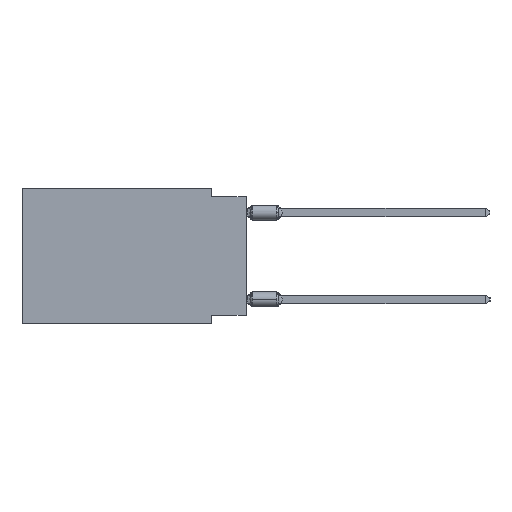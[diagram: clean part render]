
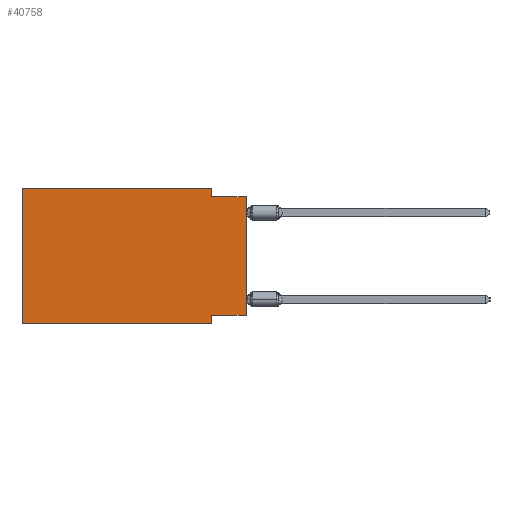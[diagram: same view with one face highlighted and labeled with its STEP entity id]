
A CAD part, left-side view. The second image highlights one B-rep face of the part: STEP entity #40758.
In plain terms, the highlighted planar face has unit normal (-1, 0, 0).
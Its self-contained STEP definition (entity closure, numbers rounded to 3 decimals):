
#18 = CARTESIAN_POINT ( 'NONE',  ( 0., 16.383, 0. ) ) ;
#158 = ORIENTED_EDGE ( 'NONE', *, *, #26595, .F. ) ;
#1688 = VERTEX_POINT ( 'NONE', #26304 ) ;
#2067 = ORIENTED_EDGE ( 'NONE', *, *, #7733, .T. ) ;
#2232 = VECTOR ( 'NONE', #34765, 1000. ) ;
#2421 = DIRECTION ( 'NONE',  ( 0., 0., -1. ) ) ;
#3027 = LINE ( 'NONE', #21885, #21431 ) ;
#3165 = CARTESIAN_POINT ( 'NONE',  ( 0., 2.54, 0. ) ) ;
#3428 = CARTESIAN_POINT ( 'NONE',  ( 0., 0., -0.635 ) ) ;
#3442 = CARTESIAN_POINT ( 'NONE',  ( 0., 0., -9.271 ) ) ;
#4793 = DIRECTION ( 'NONE',  ( 0., 0., -1. ) ) ;
#5725 = FACE_OUTER_BOUND ( 'NONE', #12027, .T. ) ;
#5744 = LINE ( 'NONE', #18407, #35977 ) ;
#6057 = VERTEX_POINT ( 'NONE', #3428 ) ;
#6160 = VERTEX_POINT ( 'NONE', #10678 ) ;
#6888 = ORIENTED_EDGE ( 'NONE', *, *, #25334, .F. ) ;
#7541 = DIRECTION ( 'NONE',  ( 0., 0., 1. ) ) ;
#7733 = EDGE_CURVE ( 'NONE', #6160, #6057, #5744, .T. ) ;
#7783 = VERTEX_POINT ( 'NONE', #19627 ) ;
#8869 = DIRECTION ( 'NONE',  ( 0., 0., 1. ) ) ;
#9450 = LINE ( 'NONE', #3442, #2232 ) ;
#9668 = DIRECTION ( 'NONE',  ( 0., -1., 0. ) ) ;
#10678 = CARTESIAN_POINT ( 'NONE',  ( 0., 0., -9.271 ) ) ;
#10879 = LINE ( 'NONE', #32650, #23352 ) ;
#11966 = CARTESIAN_POINT ( 'NONE',  ( 0., 16.383, 0. ) ) ;
#12027 = EDGE_LOOP ( 'NONE', ( #2067, #26574, #6888, #27103, #158, #29478, #27595, #31721 ) ) ;
#14845 = EDGE_CURVE ( 'NONE', #1688, #39297, #36729, .T. ) ;
#15469 = DIRECTION ( 'NONE',  ( 1., 0., 0. ) ) ;
#16641 = DIRECTION ( 'NONE',  ( 0., 0., -1. ) ) ;
#18407 = CARTESIAN_POINT ( 'NONE',  ( 0., 0., 0. ) ) ;
#19126 = VECTOR ( 'NONE', #4793, 1000. ) ;
#19368 = CARTESIAN_POINT ( 'NONE',  ( 0., 16.383, 0. ) ) ;
#19627 = CARTESIAN_POINT ( 'NONE',  ( 0., 2.54, 0. ) ) ;
#21431 = VECTOR ( 'NONE', #9668, 1000. ) ;
#21869 = CARTESIAN_POINT ( 'NONE',  ( 0., 16.383, -9.906 ) ) ;
#21885 = CARTESIAN_POINT ( 'NONE',  ( 0., 16.383, 0. ) ) ;
#23114 = DIRECTION ( 'NONE',  ( 0., -1., 0. ) ) ;
#23352 = VECTOR ( 'NONE', #23114, 1000. ) ;
#25334 = EDGE_CURVE ( 'NONE', #7783, #39717, #34690, .T. ) ;
#26304 = CARTESIAN_POINT ( 'NONE',  ( 0., 2.54, -9.271 ) ) ;
#26574 = ORIENTED_EDGE ( 'NONE', *, *, #38505, .F. ) ;
#26595 = EDGE_CURVE ( 'NONE', #27610, #29592, #35954, .T. ) ;
#27103 = ORIENTED_EDGE ( 'NONE', *, *, #30941, .F. ) ;
#27140 = VECTOR ( 'NONE', #16641, 1000. ) ;
#27595 = ORIENTED_EDGE ( 'NONE', *, *, #14845, .F. ) ;
#27610 = VERTEX_POINT ( 'NONE', #21869 ) ;
#28966 = LINE ( 'NONE', #34977, #34037 ) ;
#29478 = ORIENTED_EDGE ( 'NONE', *, *, #40991, .T. ) ;
#29592 = VERTEX_POINT ( 'NONE', #18 ) ;
#30941 = EDGE_CURVE ( 'NONE', #29592, #7783, #3027, .T. ) ;
#31065 = EDGE_CURVE ( 'NONE', #6160, #1688, #9450, .T. ) ;
#31721 = ORIENTED_EDGE ( 'NONE', *, *, #31065, .F. ) ;
#32049 = CARTESIAN_POINT ( 'NONE',  ( 0., 2.54, -0.635 ) ) ;
#32650 = CARTESIAN_POINT ( 'NONE',  ( 0., 0., -0.635 ) ) ;
#33002 = CARTESIAN_POINT ( 'NONE',  ( 0., 2.54, -9.906 ) ) ;
#33323 = CARTESIAN_POINT ( 'NONE',  ( 0., 2.54, -9.906 ) ) ;
#34037 = VECTOR ( 'NONE', #37861, 1000. ) ;
#34690 = LINE ( 'NONE', #3165, #27140 ) ;
#34765 = DIRECTION ( 'NONE',  ( 0., 1., 0. ) ) ;
#34977 = CARTESIAN_POINT ( 'NONE',  ( 0., 16.383, -9.906 ) ) ;
#35954 = LINE ( 'NONE', #19368, #39113 ) ;
#35977 = VECTOR ( 'NONE', #8869, 1000. ) ;
#36729 = LINE ( 'NONE', #33002, #19126 ) ;
#37861 = DIRECTION ( 'NONE',  ( 0., -1., 0. ) ) ;
#37973 = AXIS2_PLACEMENT_3D ( 'NONE', #11966, #15469, #2421 ) ;
#38505 = EDGE_CURVE ( 'NONE', #39717, #6057, #10879, .T. ) ;
#39113 = VECTOR ( 'NONE', #7541, 1000. ) ;
#39297 = VERTEX_POINT ( 'NONE', #33323 ) ;
#39717 = VERTEX_POINT ( 'NONE', #32049 ) ;
#40158 = PLANE ( 'NONE',  #37973 ) ;
#40758 = ADVANCED_FACE ( 'NONE', ( #5725 ), #40158, .F. ) ;
#40991 = EDGE_CURVE ( 'NONE', #27610, #39297, #28966, .T. ) ;
